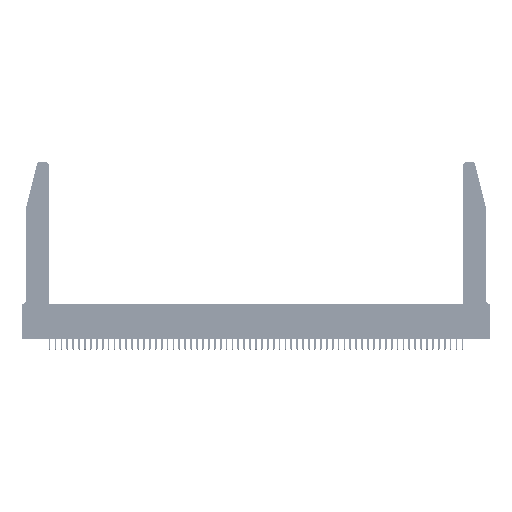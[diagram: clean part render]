
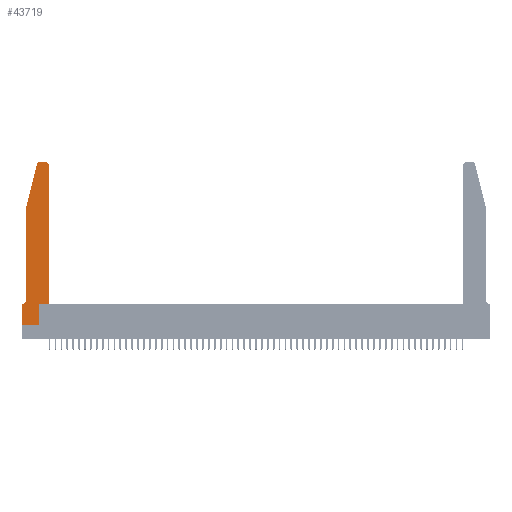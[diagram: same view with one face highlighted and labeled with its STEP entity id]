
A CAD part, top view. The second image highlights one B-rep face of the part: STEP entity #43719.
In plain terms, the highlighted planar face has unit normal (0, 0, 1).
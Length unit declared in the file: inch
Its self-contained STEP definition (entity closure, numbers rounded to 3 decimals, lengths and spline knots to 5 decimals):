
#412 = ORIENTED_EDGE ( 'NONE', *, *, #40758, .T. ) ;
#611 = CARTESIAN_POINT ( 'NONE',  ( 0.4205, 2.75, 0.37 ) ) ;
#862 = VERTEX_POINT ( 'NONE', #30162 ) ;
#1818 = EDGE_CURVE ( 'NONE', #862, #54774, #26116, .T. ) ;
#2153 = DIRECTION ( 'NONE',  ( 0., 0., 1. ) ) ;
#2980 = ORIENTED_EDGE ( 'NONE', *, *, #33481, .T. ) ;
#3090 = CARTESIAN_POINT ( 'NONE',  ( 0.2865, 0.35, 0.37 ) ) ;
#4168 = ORIENTED_EDGE ( 'NONE', *, *, #25014, .T. ) ;
#4262 = CARTESIAN_POINT ( 'NONE',  ( 0.4505, 0.35, 0.37 ) ) ;
#5023 = CARTESIAN_POINT ( 'NONE',  ( 0.0755, 0.42, 0.37 ) ) ;
#5904 = ORIENTED_EDGE ( 'NONE', *, *, #27021, .T. ) ;
#6808 = CARTESIAN_POINT ( 'NONE',  ( 0.2865, 0.35, 0.37 ) ) ;
#7077 = EDGE_CURVE ( 'NONE', #7607, #53195, #30290, .T. ) ;
#7607 = VERTEX_POINT ( 'NONE', #6808 ) ;
#8372 = VECTOR ( 'NONE', #42639, 39.37008 ) ;
#10083 = CARTESIAN_POINT ( 'NONE',  ( 0.0055, 0.35, 0.37 ) ) ;
#11312 = LINE ( 'NONE', #22656, #34680 ) ;
#12691 = EDGE_CURVE ( 'NONE', #55298, #862, #43341, .T. ) ;
#14432 = ORIENTED_EDGE ( 'NONE', *, *, #17166, .T. ) ;
#14654 = ORIENTED_EDGE ( 'NONE', *, *, #15720, .T. ) ;
#15217 = CARTESIAN_POINT ( 'NONE',  ( 0.0755, 0.35, 0.37 ) ) ;
#15343 = AXIS2_PLACEMENT_3D ( 'NONE', #46611, #20365, #50987 ) ;
#15631 = CARTESIAN_POINT ( 'NONE',  ( 0.2865, 0., 0.37 ) ) ;
#15720 = EDGE_CURVE ( 'NONE', #53195, #23108, #54296, .T. ) ;
#16233 = DIRECTION ( 'NONE',  ( 1., 0., 0. ) ) ;
#16386 = CARTESIAN_POINT ( 'NONE',  ( 0., 0., 0.37 ) ) ;
#16508 = CIRCLE ( 'NONE', #41988, 0.03 ) ;
#16613 = LINE ( 'NONE', #15217, #26912 ) ;
#17166 = EDGE_CURVE ( 'NONE', #40362, #41147, #16508, .T. ) ;
#17619 = VERTEX_POINT ( 'NONE', #5023 ) ;
#17794 = DIRECTION ( 'NONE',  ( 0., 1., 0. ) ) ;
#18268 = ORIENTED_EDGE ( 'NONE', *, *, #37750, .T. ) ;
#18345 = DIRECTION ( 'NONE',  ( 0., 0., -1. ) ) ;
#19017 = PLANE ( 'NONE',  #38891 ) ;
#20365 = DIRECTION ( 'NONE',  ( 0., 0., 1. ) ) ;
#22656 = CARTESIAN_POINT ( 'NONE',  ( 0.2605, 2.75, 0.37 ) ) ;
#23108 = VERTEX_POINT ( 'NONE', #25236 ) ;
#23219 = DIRECTION ( 'NONE',  ( 0., 0., 1. ) ) ;
#23417 = DIRECTION ( 'NONE',  ( 1., 0., 0. ) ) ;
#24246 = CARTESIAN_POINT ( 'NONE',  ( 0.0755, 2., 0.37 ) ) ;
#24448 = DIRECTION ( 'NONE',  ( -0.239, -0.971, 0. ) ) ;
#24888 = VERTEX_POINT ( 'NONE', #10083 ) ;
#25014 = EDGE_CURVE ( 'NONE', #41147, #37430, #54859, .T. ) ;
#25236 = CARTESIAN_POINT ( 'NONE',  ( 0.4505, 2.72, 0.37 ) ) ;
#26116 = LINE ( 'NONE', #47638, #37781 ) ;
#26449 = FACE_OUTER_BOUND ( 'NONE', #48533, .T. ) ;
#26912 = VECTOR ( 'NONE', #32673, 39.37008 ) ;
#27021 = EDGE_CURVE ( 'NONE', #23108, #42334, #56665, .T. ) ;
#28477 = CARTESIAN_POINT ( 'NONE',  ( 0.284, 2.72, 0.37 ) ) ;
#30162 = CARTESIAN_POINT ( 'NONE',  ( 0., 0., 0.37 ) ) ;
#30290 = LINE ( 'NONE', #51262, #41914 ) ;
#30305 = VECTOR ( 'NONE', #55747, 39.37008 ) ;
#30867 = CARTESIAN_POINT ( 'NONE',  ( 0.4505, 0.35, 0.37 ) ) ;
#31688 = CIRCLE ( 'NONE', #48580, 0.07 ) ;
#32673 = DIRECTION ( 'NONE',  ( -1., 0., 0. ) ) ;
#32896 = DIRECTION ( 'NONE',  ( 1., 0., 0. ) ) ;
#33481 = EDGE_CURVE ( 'NONE', #17619, #24888, #31688, .T. ) ;
#34413 = VECTOR ( 'NONE', #24448, 39.37008 ) ;
#34509 = ORIENTED_EDGE ( 'NONE', *, *, #1818, .T. ) ;
#34680 = VECTOR ( 'NONE', #40107, 39.37008 ) ;
#34906 = ORIENTED_EDGE ( 'NONE', *, *, #50972, .T. ) ;
#37430 = VERTEX_POINT ( 'NONE', #53612 ) ;
#37750 = EDGE_CURVE ( 'NONE', #37430, #17619, #51215, .T. ) ;
#37781 = VECTOR ( 'NONE', #52001, 39.37008 ) ;
#38176 = CARTESIAN_POINT ( 'NONE',  ( 0.284, 2.75, 0.37 ) ) ;
#38891 = AXIS2_PLACEMENT_3D ( 'NONE', #40859, #23219, #23417 ) ;
#39612 = VECTOR ( 'NONE', #46282, 39.37008 ) ;
#40107 = DIRECTION ( 'NONE',  ( -1., 0., 0. ) ) ;
#40362 = VERTEX_POINT ( 'NONE', #38176 ) ;
#40705 = CARTESIAN_POINT ( 'NONE',  ( 0., 0.35, 0.37 ) ) ;
#40758 = EDGE_CURVE ( 'NONE', #24888, #55298, #16613, .T. ) ;
#40859 = CARTESIAN_POINT ( 'NONE',  ( 0., 0.35, 0.37 ) ) ;
#41147 = VERTEX_POINT ( 'NONE', #44712 ) ;
#41914 = VECTOR ( 'NONE', #16233, 39.37008 ) ;
#41988 = AXIS2_PLACEMENT_3D ( 'NONE', #28477, #2153, #32896 ) ;
#42334 = VERTEX_POINT ( 'NONE', #611 ) ;
#42639 = DIRECTION ( 'NONE',  ( 0., -1., 0. ) ) ;
#42746 = VECTOR ( 'NONE', #17794, 39.37008 ) ;
#43341 = LINE ( 'NONE', #16386, #8372 ) ;
#43513 = ORIENTED_EDGE ( 'NONE', *, *, #47879, .T. ) ;
#43719 = ADVANCED_FACE ( 'NONE', ( #26449 ), #19017, .T. ) ;
#44626 = CARTESIAN_POINT ( 'NONE',  ( 0.0055, 0.42, 0.37 ) ) ;
#44712 = CARTESIAN_POINT ( 'NONE',  ( 0.25487, 2.72718, 0.37 ) ) ;
#46273 = ORIENTED_EDGE ( 'NONE', *, *, #12691, .T. ) ;
#46282 = DIRECTION ( 'NONE',  ( 0., -1., 0. ) ) ;
#46611 = CARTESIAN_POINT ( 'NONE',  ( 0.4205, 2.72, 0.37 ) ) ;
#47638 = CARTESIAN_POINT ( 'NONE',  ( 0., 0., 0.37 ) ) ;
#47879 = EDGE_CURVE ( 'NONE', #42334, #40362, #11312, .T. ) ;
#48533 = EDGE_LOOP ( 'NONE', ( #43513, #14432, #4168, #18268, #2980, #412, #46273, #34509, #34906, #51953, #14654, #5904 ) ) ;
#48580 = AXIS2_PLACEMENT_3D ( 'NONE', #44626, #18345, #48989 ) ;
#48989 = DIRECTION ( 'NONE',  ( -1., 0., 0. ) ) ;
#50972 = EDGE_CURVE ( 'NONE', #54774, #7607, #53514, .T. ) ;
#50987 = DIRECTION ( 'NONE',  ( 1., 0., 0. ) ) ;
#51215 = LINE ( 'NONE', #24246, #39612 ) ;
#51262 = CARTESIAN_POINT ( 'NONE',  ( 0.4505, 0.35, 0.37 ) ) ;
#51953 = ORIENTED_EDGE ( 'NONE', *, *, #7077, .T. ) ;
#52001 = DIRECTION ( 'NONE',  ( 1., 0., 0. ) ) ;
#53195 = VERTEX_POINT ( 'NONE', #4262 ) ;
#53514 = LINE ( 'NONE', #3090, #30305 ) ;
#53612 = CARTESIAN_POINT ( 'NONE',  ( 0.0755, 2., 0.37 ) ) ;
#54296 = LINE ( 'NONE', #30867, #42746 ) ;
#54774 = VERTEX_POINT ( 'NONE', #15631 ) ;
#54859 = LINE ( 'NONE', #54997, #34413 ) ;
#54997 = CARTESIAN_POINT ( 'NONE',  ( 0.0755, 2., 0.37 ) ) ;
#55298 = VERTEX_POINT ( 'NONE', #40705 ) ;
#55747 = DIRECTION ( 'NONE',  ( 0., 1., 0. ) ) ;
#56665 = CIRCLE ( 'NONE', #15343, 0.03 ) ;
